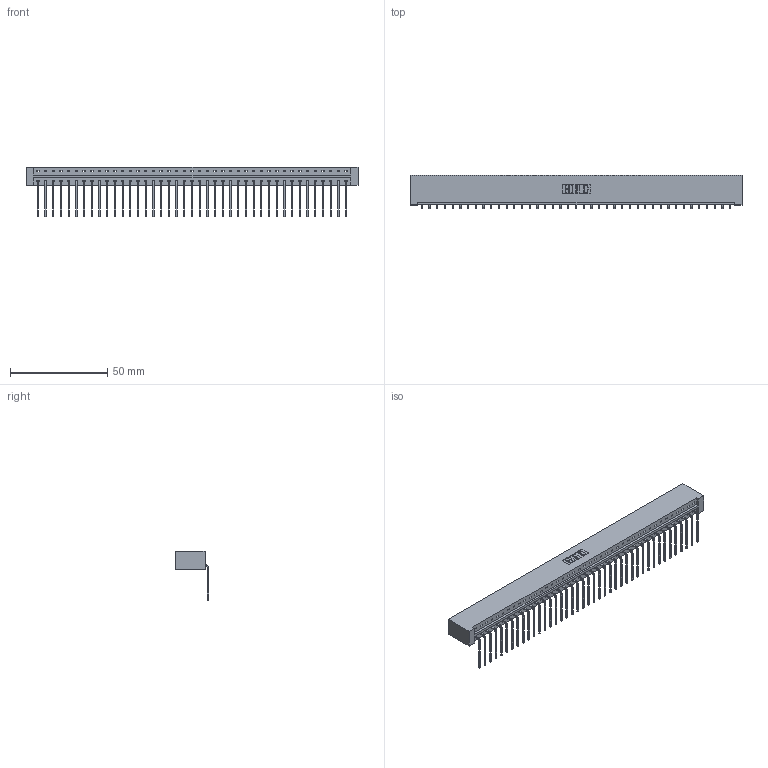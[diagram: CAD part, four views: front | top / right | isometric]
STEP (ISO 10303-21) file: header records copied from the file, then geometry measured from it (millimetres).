
FILE_DESCRIPTION (( 'STEP AP203' ), '1' );
FILE_NAME ('333-041-559-101.STEP', '2018-08-03T15:48:38', ( '' ), ( '' ), 'SwSTEP 2.0', 'SolidWorks 2016', '' );
FILE_SCHEMA (( 'CONFIG_CONTROL_DESIGN' ));
Length unit declared in the file: inch
Products named in the file (3): 333 Part_Lugless; 345-292-001_558 559 Tail - 1; 333-041-559-101
Assembly tree (42 placements, depth 2):
  333-041-559-101
    333 Part_Lugless
    345-292-001_558 559 Tail - 1  x41
Bounding box: 170.71 x 17.09 x 25.53 mm (x, y, z)
Volume: 17919.3 mm3; surface area: 20176.1 mm2
Topology: 42 solids, 42 shells, 2566 faces, 7749 edges, 5110 vertices
Faces by surface type: plane 1870, cylinder 696
Entity records: 25001 total; most frequent: CARTESIAN_POINT 4321, ORIENTED_EDGE 4298, DIRECTION 3639, EDGE_CURVE 2149, VECTOR 2029, LINE 2029, VERTEX_POINT 1430, AXIS2_PLACEMENT_3D 805
